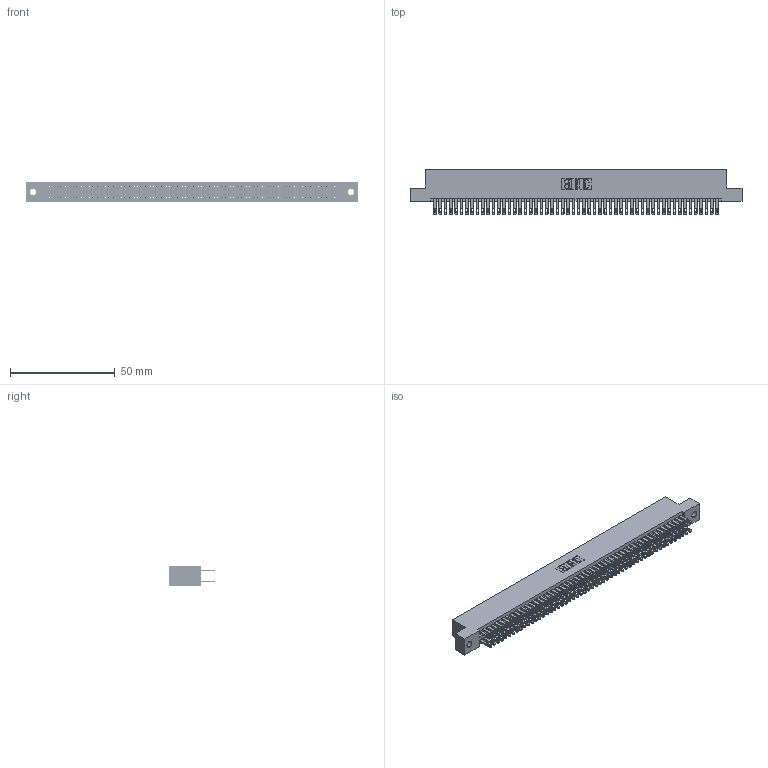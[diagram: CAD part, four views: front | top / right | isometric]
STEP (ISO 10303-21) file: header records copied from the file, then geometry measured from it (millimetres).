
FILE_DESCRIPTION (( 'STEP AP203' ), '1' );
FILE_NAME ('345-108-500-202.STEP', '2019-11-03T18:37:29', ( '' ), ( '' ), 'SwSTEP 2.0', 'SolidWorks 2016', '' );
FILE_SCHEMA (( 'CONFIG_CONTROL_DESIGN' ));
Length unit declared in the file: inch
Products named in the file (3): 345-108-500-202; 345 Part_Flush Mounting Lugs - 0.128 Dia; 345-292-001_345-293-100
Assembly tree (109 placements, depth 2):
  345-108-500-202
    345 Part_Flush Mounting Lugs - 0.128 Dia
    345-292-001_345-293-100  x108
Bounding box: 158.37 x 21.51 x 9.4 mm (x, y, z)
Volume: 15788.9 mm3; surface area: 24399.8 mm2
Topology: 109 solids, 109 shells, 5094 faces, 15569 edges, 10378 vertices
Faces by surface type: plane 2996, cylinder 2098
Entity records: 40687 total; most frequent: CARTESIAN_POINT 6808, ORIENTED_EDGE 6742, DIRECTION 5991, EDGE_CURVE 3371, LINE 3019, VECTOR 3019, VERTEX_POINT 2246, AXIS2_PLACEMENT_3D 1486
